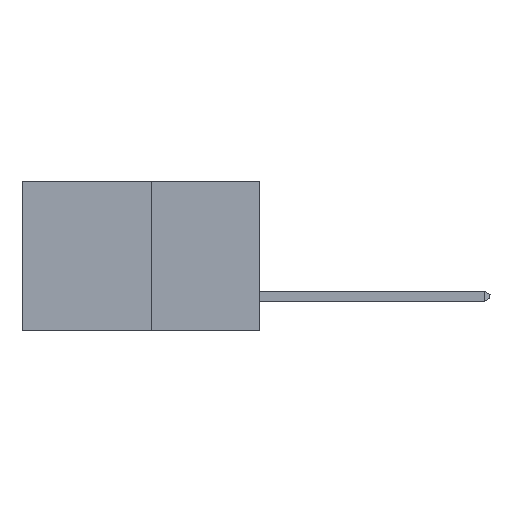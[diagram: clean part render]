
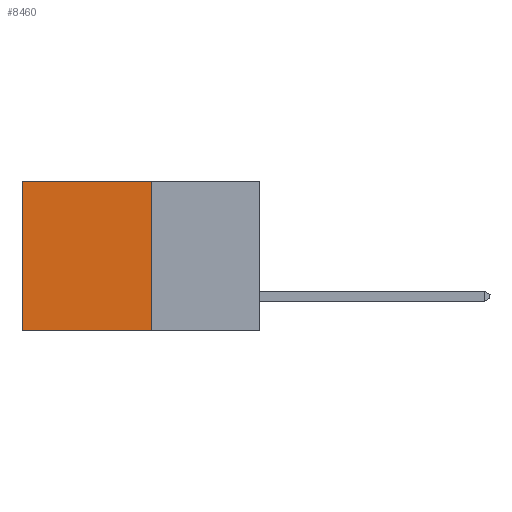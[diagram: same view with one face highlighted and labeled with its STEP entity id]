
A CAD part, left-side view. The second image highlights one B-rep face of the part: STEP entity #8460.
In plain terms, the highlighted planar face has unit normal (-1, 0, 0).
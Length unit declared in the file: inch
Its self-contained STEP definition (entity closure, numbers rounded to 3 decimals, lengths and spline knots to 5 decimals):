
#362 = LINE ( 'NONE', #4029, #19486 ) ;
#495 = DIRECTION ( 'NONE',  ( 0., 1., 0. ) ) ;
#809 = EDGE_CURVE ( 'NONE', #3645, #19391, #11735, .T. ) ;
#2707 = EDGE_LOOP ( 'NONE', ( #9608, #4763, #8452, #7279 ) ) ;
#3645 = VERTEX_POINT ( 'NONE', #15076 ) ;
#3652 = LINE ( 'NONE', #6654, #15675 ) ;
#4029 = CARTESIAN_POINT ( 'NONE',  ( 0.277, 0.59, -0.37 ) ) ;
#4763 = ORIENTED_EDGE ( 'NONE', *, *, #809, .F. ) ;
#5481 = DIRECTION ( 'NONE',  ( 0., 0., -1. ) ) ;
#6654 = CARTESIAN_POINT ( 'NONE',  ( 0.277, 0.27, 0. ) ) ;
#7279 = ORIENTED_EDGE ( 'NONE', *, *, #19267, .T. ) ;
#7411 = PLANE ( 'NONE',  #16645 ) ;
#8452 = ORIENTED_EDGE ( 'NONE', *, *, #10243, .F. ) ;
#8460 = ADVANCED_FACE ( 'NONE', ( #19454 ), #7411, .F. ) ;
#8733 = VERTEX_POINT ( 'NONE', #12497 ) ;
#9608 = ORIENTED_EDGE ( 'NONE', *, *, #16696, .T. ) ;
#10053 = DIRECTION ( 'NONE',  ( 0., 0., -1. ) ) ;
#10125 = CARTESIAN_POINT ( 'NONE',  ( 0.277, 0.59, 0. ) ) ;
#10243 = EDGE_CURVE ( 'NONE', #8733, #3645, #17531, .T. ) ;
#10443 = DIRECTION ( 'NONE',  ( 0., 0., -1. ) ) ;
#11735 = LINE ( 'NONE', #12675, #15253 ) ;
#12497 = CARTESIAN_POINT ( 'NONE',  ( 0.277, 0.27, 0. ) ) ;
#12675 = CARTESIAN_POINT ( 'NONE',  ( 0.277, 0.27, -0.37 ) ) ;
#12960 = CARTESIAN_POINT ( 'NONE',  ( 0.277, 0.27, -0.37 ) ) ;
#13005 = CARTESIAN_POINT ( 'NONE',  ( 0.277, 0.59, -0.37 ) ) ;
#13526 = VECTOR ( 'NONE', #5481, 39.37008 ) ;
#14868 = DIRECTION ( 'NONE',  ( 0., 1., 0. ) ) ;
#15076 = CARTESIAN_POINT ( 'NONE',  ( 0.277, 0.27, -0.37 ) ) ;
#15253 = VECTOR ( 'NONE', #14868, 39.37008 ) ;
#15675 = VECTOR ( 'NONE', #495, 39.37008 ) ;
#16645 = AXIS2_PLACEMENT_3D ( 'NONE', #17923, #19384, #10443 ) ;
#16696 = EDGE_CURVE ( 'NONE', #16703, #19391, #362, .T. ) ;
#16703 = VERTEX_POINT ( 'NONE', #10125 ) ;
#17531 = LINE ( 'NONE', #12960, #13526 ) ;
#17923 = CARTESIAN_POINT ( 'NONE',  ( 0.277, 0.27, -0.37 ) ) ;
#19267 = EDGE_CURVE ( 'NONE', #8733, #16703, #3652, .T. ) ;
#19384 = DIRECTION ( 'NONE',  ( 1., 0., 0. ) ) ;
#19391 = VERTEX_POINT ( 'NONE', #13005 ) ;
#19454 = FACE_OUTER_BOUND ( 'NONE', #2707, .T. ) ;
#19486 = VECTOR ( 'NONE', #10053, 39.37008 ) ;
